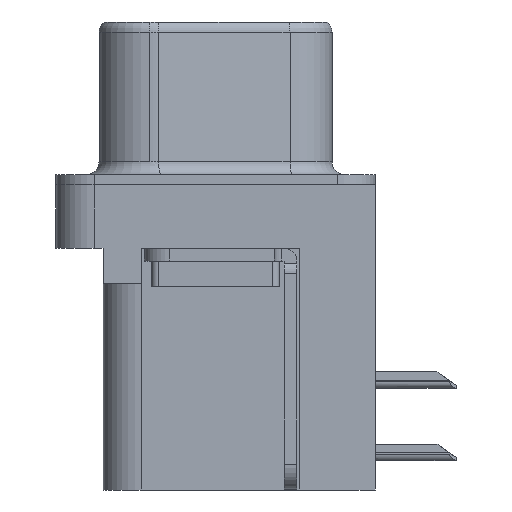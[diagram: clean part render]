
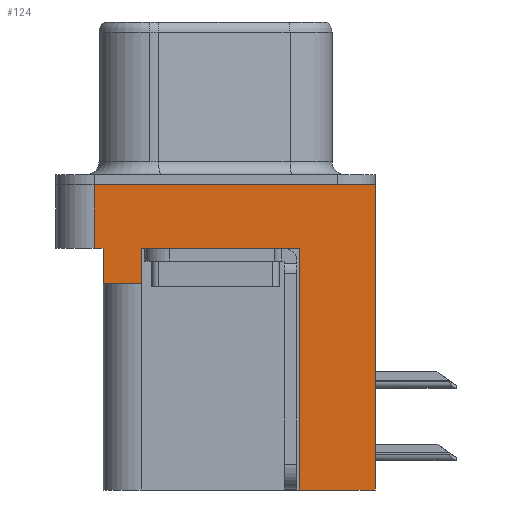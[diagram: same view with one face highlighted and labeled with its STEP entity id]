
A CAD part, left-side view. The second image highlights one B-rep face of the part: STEP entity #124.
In plain terms, the highlighted planar face has unit normal (-1, 0, 0).
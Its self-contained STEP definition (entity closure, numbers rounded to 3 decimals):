
#121 = CARTESIAN_POINT ( 'NONE',  ( -3., -6.275, -12. ) ) ;
#124 = ADVANCED_FACE ( 'NONE', ( #4416 ), #12814, .T. ) ;
#155 = VERTEX_POINT ( 'NONE', #4476 ) ;
#223 = CARTESIAN_POINT ( 'NONE',  ( -3., -3.295, -12. ) ) ;
#283 = DIRECTION ( 'NONE',  ( 0., 0., 1. ) ) ;
#805 = LINE ( 'NONE', #12027, #5718 ) ;
#1448 = AXIS2_PLACEMENT_3D ( 'NONE', #16264, #11153, #2792 ) ;
#1752 = DIRECTION ( 'NONE',  ( 0., 0., 1. ) ) ;
#2188 = EDGE_CURVE ( 'NONE', #20473, #19859, #6343, .T. ) ;
#2245 = LINE ( 'NONE', #13892, #6269 ) ;
#2251 = EDGE_CURVE ( 'NONE', #21592, #155, #3907, .T. ) ;
#2792 = DIRECTION ( 'NONE',  ( 0., 0., 1. ) ) ;
#3195 = CARTESIAN_POINT ( 'NONE',  ( -3., 2.895, -2.5 ) ) ;
#3344 = EDGE_CURVE ( 'NONE', #4105, #155, #2245, .T. ) ;
#3592 = LINE ( 'NONE', #12093, #21255 ) ;
#3791 = ORIENTED_EDGE ( 'NONE', *, *, #16158, .F. ) ;
#3800 = DIRECTION ( 'NONE',  ( 0., 0., 1. ) ) ;
#3907 = LINE ( 'NONE', #6433, #8957 ) ;
#4105 = VERTEX_POINT ( 'NONE', #121 ) ;
#4416 = FACE_OUTER_BOUND ( 'NONE', #11461, .T. ) ;
#4476 = CARTESIAN_POINT ( 'NONE',  ( -3., -6.275, 0. ) ) ;
#4524 = DIRECTION ( 'NONE',  ( 0., 0., 1. ) ) ;
#4696 = EDGE_CURVE ( 'NONE', #12646, #12076, #12857, .T. ) ;
#5380 = DIRECTION ( 'NONE',  ( 0., -1., 0. ) ) ;
#5718 = VECTOR ( 'NONE', #1752, 1000. ) ;
#5890 = CARTESIAN_POINT ( 'NONE',  ( -3., 4.775, -2.5 ) ) ;
#6181 = EDGE_CURVE ( 'NONE', #20473, #12646, #9304, .T. ) ;
#6269 = VECTOR ( 'NONE', #3800, 1000. ) ;
#6343 = LINE ( 'NONE', #16607, #19994 ) ;
#6433 = CARTESIAN_POINT ( 'NONE',  ( -3., -6.275, 0. ) ) ;
#7230 = CARTESIAN_POINT ( 'NONE',  ( -3., 4.425, -3.9 ) ) ;
#7245 = LINE ( 'NONE', #18194, #12349 ) ;
#7961 = VECTOR ( 'NONE', #5380, 1000. ) ;
#7974 = CARTESIAN_POINT ( 'NONE',  ( -3., 2.895, -3.9 ) ) ;
#8870 = EDGE_CURVE ( 'NONE', #4105, #10884, #16375, .T. ) ;
#8957 = VECTOR ( 'NONE', #14821, 1000. ) ;
#9304 = LINE ( 'NONE', #16398, #17900 ) ;
#10135 = VERTEX_POINT ( 'NONE', #11538 ) ;
#10815 = EDGE_CURVE ( 'NONE', #19859, #10135, #11986, .T. ) ;
#10884 = VERTEX_POINT ( 'NONE', #20972 ) ;
#11153 = DIRECTION ( 'NONE',  ( -1., 0., 0. ) ) ;
#11236 = ORIENTED_EDGE ( 'NONE', *, *, #8870, .F. ) ;
#11461 = EDGE_LOOP ( 'NONE', ( #13807, #3791, #13010, #12816, #17173, #14258, #17450, #22220, #11236, #21578 ) ) ;
#11538 = CARTESIAN_POINT ( 'NONE',  ( -3., -3.295, -2.5 ) ) ;
#11986 = LINE ( 'NONE', #13531, #7961 ) ;
#12027 = CARTESIAN_POINT ( 'NONE',  ( -3., -3.295, -12. ) ) ;
#12076 = VERTEX_POINT ( 'NONE', #17350 ) ;
#12093 = CARTESIAN_POINT ( 'NONE',  ( -3., 4.775, -2.5 ) ) ;
#12349 = VECTOR ( 'NONE', #14580, 1000. ) ;
#12646 = VERTEX_POINT ( 'NONE', #20300 ) ;
#12814 = PLANE ( 'NONE',  #1448 ) ;
#12816 = ORIENTED_EDGE ( 'NONE', *, *, #4696, .F. ) ;
#12857 = LINE ( 'NONE', #7230, #16346 ) ;
#13010 = ORIENTED_EDGE ( 'NONE', *, *, #20439, .T. ) ;
#13531 = CARTESIAN_POINT ( 'NONE',  ( -3., -6.275, -2.5 ) ) ;
#13807 = ORIENTED_EDGE ( 'NONE', *, *, #2251, .F. ) ;
#13892 = CARTESIAN_POINT ( 'NONE',  ( -3., -6.275, -2.5 ) ) ;
#14258 = ORIENTED_EDGE ( 'NONE', *, *, #2188, .T. ) ;
#14580 = DIRECTION ( 'NONE',  ( 0., -1., 0. ) ) ;
#14821 = DIRECTION ( 'NONE',  ( 0., -1., 0. ) ) ;
#15844 = VECTOR ( 'NONE', #20939, 1000. ) ;
#16158 = EDGE_CURVE ( 'NONE', #16262, #21592, #3592, .T. ) ;
#16239 = EDGE_CURVE ( 'NONE', #10884, #10135, #805, .T. ) ;
#16262 = VERTEX_POINT ( 'NONE', #5890 ) ;
#16263 = CARTESIAN_POINT ( 'NONE',  ( -3., 4.775, 0. ) ) ;
#16264 = CARTESIAN_POINT ( 'NONE',  ( -3., -6.275, -2.5 ) ) ;
#16346 = VECTOR ( 'NONE', #17651, 1000. ) ;
#16375 = LINE ( 'NONE', #223, #15844 ) ;
#16398 = CARTESIAN_POINT ( 'NONE',  ( -3., 4.425, -3.9 ) ) ;
#16607 = CARTESIAN_POINT ( 'NONE',  ( -3., 2.895, -3.9 ) ) ;
#17173 = ORIENTED_EDGE ( 'NONE', *, *, #6181, .F. ) ;
#17350 = CARTESIAN_POINT ( 'NONE',  ( -3., 4.425, -2.5 ) ) ;
#17450 = ORIENTED_EDGE ( 'NONE', *, *, #10815, .T. ) ;
#17651 = DIRECTION ( 'NONE',  ( 0., 0., 1. ) ) ;
#17900 = VECTOR ( 'NONE', #22027, 1000. ) ;
#18194 = CARTESIAN_POINT ( 'NONE',  ( -3., -6.275, -2.5 ) ) ;
#19859 = VERTEX_POINT ( 'NONE', #3195 ) ;
#19994 = VECTOR ( 'NONE', #4524, 1000. ) ;
#20300 = CARTESIAN_POINT ( 'NONE',  ( -3., 4.425, -3.9 ) ) ;
#20439 = EDGE_CURVE ( 'NONE', #16262, #12076, #7245, .T. ) ;
#20473 = VERTEX_POINT ( 'NONE', #7974 ) ;
#20939 = DIRECTION ( 'NONE',  ( 0., 1., 0. ) ) ;
#20972 = CARTESIAN_POINT ( 'NONE',  ( -3., -3.295, -12. ) ) ;
#21255 = VECTOR ( 'NONE', #283, 1000. ) ;
#21578 = ORIENTED_EDGE ( 'NONE', *, *, #3344, .T. ) ;
#21592 = VERTEX_POINT ( 'NONE', #16263 ) ;
#22027 = DIRECTION ( 'NONE',  ( 0., 1., 0. ) ) ;
#22220 = ORIENTED_EDGE ( 'NONE', *, *, #16239, .F. ) ;
